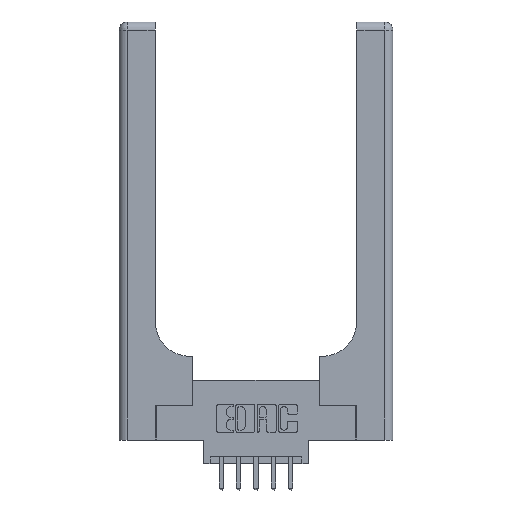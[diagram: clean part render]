
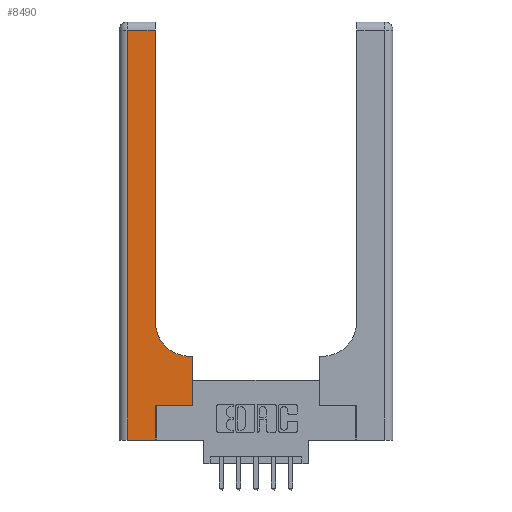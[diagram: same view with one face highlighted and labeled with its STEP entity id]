
A CAD part, top view. The second image highlights one B-rep face of the part: STEP entity #8490.
In plain terms, the highlighted planar face has unit normal (0, 0, 1).
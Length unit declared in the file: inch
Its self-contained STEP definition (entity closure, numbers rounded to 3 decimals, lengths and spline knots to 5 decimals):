
#229 = VERTEX_POINT ( 'NONE', #4516 ) ;
#264 = CARTESIAN_POINT ( 'NONE',  ( 0.265, 0., 0.37 ) ) ;
#535 = CARTESIAN_POINT ( 'NONE',  ( 0.06, 2.94, 0.37 ) ) ;
#684 = EDGE_CURVE ( 'NONE', #13759, #13767, #4708, .T. ) ;
#836 = DIRECTION ( 'NONE',  ( 0., 0., -1. ) ) ;
#930 = CARTESIAN_POINT ( 'NONE',  ( 0.26, 3., 0.37 ) ) ;
#999 = CARTESIAN_POINT ( 'NONE',  ( 0.06, 3., 0.37 ) ) ;
#1139 = VERTEX_POINT ( 'NONE', #5808 ) ;
#1253 = VECTOR ( 'NONE', #1287, 39.37008 ) ;
#1287 = DIRECTION ( 'NONE',  ( -1., 0., 0. ) ) ;
#1362 = CARTESIAN_POINT ( 'NONE',  ( 0.26, 0.6, 0.37 ) ) ;
#1393 = EDGE_CURVE ( 'NONE', #5581, #1139, #13843, .T. ) ;
#2218 = VECTOR ( 'NONE', #6443, 39.37008 ) ;
#2433 = VECTOR ( 'NONE', #2627, 39.37008 ) ;
#2560 = LINE ( 'NONE', #2629, #2978 ) ;
#2594 = LINE ( 'NONE', #6953, #7939 ) ;
#2627 = DIRECTION ( 'NONE',  ( 1., 0., 0. ) ) ;
#2629 = CARTESIAN_POINT ( 'NONE',  ( 0.528, 0.25, 0.37 ) ) ;
#2834 = VECTOR ( 'NONE', #10107, 39.37008 ) ;
#2870 = ORIENTED_EDGE ( 'NONE', *, *, #9795, .T. ) ;
#2978 = VECTOR ( 'NONE', #4777, 39.37008 ) ;
#3374 = VECTOR ( 'NONE', #12914, 39.37008 ) ;
#3708 = CARTESIAN_POINT ( 'NONE',  ( 0.265, 0.25, 0.37 ) ) ;
#4143 = CARTESIAN_POINT ( 'NONE',  ( 0.51, 0.85, 0.37 ) ) ;
#4402 = CARTESIAN_POINT ( 'NONE',  ( 0., 0., 0.37 ) ) ;
#4435 = CARTESIAN_POINT ( 'NONE',  ( 0., 3., 0.37 ) ) ;
#4464 = LINE ( 'NONE', #4402, #10643 ) ;
#4466 = CARTESIAN_POINT ( 'NONE',  ( 0.26, 2.94, 0.37 ) ) ;
#4516 = CARTESIAN_POINT ( 'NONE',  ( 0.528, 0.25, 0.37 ) ) ;
#4708 = LINE ( 'NONE', #1362, #1253 ) ;
#4777 = DIRECTION ( 'NONE',  ( 0., 1., 0. ) ) ;
#5541 = CARTESIAN_POINT ( 'NONE',  ( 0.51, 0.6, 0.37 ) ) ;
#5581 = VERTEX_POINT ( 'NONE', #8639 ) ;
#5808 = CARTESIAN_POINT ( 'NONE',  ( 0.265, 0.25, 0.37 ) ) ;
#6438 = PLANE ( 'NONE',  #11769 ) ;
#6443 = DIRECTION ( 'NONE',  ( 0., 1., 0. ) ) ;
#6792 = AXIS2_PLACEMENT_3D ( 'NONE', #4143, #836, #13835 ) ;
#6953 = CARTESIAN_POINT ( 'NONE',  ( 0., 2.94, 0.37 ) ) ;
#7097 = DIRECTION ( 'NONE',  ( -1., 0., 0. ) ) ;
#7404 = ORIENTED_EDGE ( 'NONE', *, *, #1393, .T. ) ;
#7445 = CIRCLE ( 'NONE', #6792, 0.25 ) ;
#7471 = EDGE_CURVE ( 'NONE', #1139, #229, #13470, .T. ) ;
#7489 = EDGE_CURVE ( 'NONE', #13767, #8089, #7445, .T. ) ;
#7701 = FACE_OUTER_BOUND ( 'NONE', #12515, .T. ) ;
#7719 = CARTESIAN_POINT ( 'NONE',  ( 0.528, 0.6, 0.37 ) ) ;
#7931 = ORIENTED_EDGE ( 'NONE', *, *, #10872, .T. ) ;
#7939 = VECTOR ( 'NONE', #7097, 39.37008 ) ;
#8089 = VERTEX_POINT ( 'NONE', #13291 ) ;
#8354 = VERTEX_POINT ( 'NONE', #9433 ) ;
#8490 = ADVANCED_FACE ( 'NONE', ( #7701 ), #6438, .F. ) ;
#8639 = CARTESIAN_POINT ( 'NONE',  ( 0.265, 0., 0.37 ) ) ;
#8767 = DIRECTION ( 'NONE',  ( 0., 0., -1. ) ) ;
#8933 = ORIENTED_EDGE ( 'NONE', *, *, #7471, .T. ) ;
#9433 = CARTESIAN_POINT ( 'NONE',  ( 0.06, 0., 0.37 ) ) ;
#9557 = EDGE_CURVE ( 'NONE', #8354, #5581, #4464, .T. ) ;
#9767 = LINE ( 'NONE', #930, #2218 ) ;
#9792 = EDGE_CURVE ( 'NONE', #8089, #13301, #9767, .T. ) ;
#9795 = EDGE_CURVE ( 'NONE', #10459, #8354, #9839, .T. ) ;
#9839 = LINE ( 'NONE', #999, #3374 ) ;
#9863 = ORIENTED_EDGE ( 'NONE', *, *, #9792, .T. ) ;
#10107 = DIRECTION ( 'NONE',  ( 0., 1., 0. ) ) ;
#10459 = VERTEX_POINT ( 'NONE', #535 ) ;
#10643 = VECTOR ( 'NONE', #12414, 39.37008 ) ;
#10872 = EDGE_CURVE ( 'NONE', #13301, #10459, #2594, .T. ) ;
#10958 = ORIENTED_EDGE ( 'NONE', *, *, #684, .T. ) ;
#11683 = ORIENTED_EDGE ( 'NONE', *, *, #9557, .T. ) ;
#11769 = AXIS2_PLACEMENT_3D ( 'NONE', #4435, #8767, #13989 ) ;
#12076 = ORIENTED_EDGE ( 'NONE', *, *, #7489, .T. ) ;
#12414 = DIRECTION ( 'NONE',  ( 1., 0., 0. ) ) ;
#12502 = EDGE_CURVE ( 'NONE', #229, #13759, #2560, .T. ) ;
#12515 = EDGE_LOOP ( 'NONE', ( #9863, #7931, #2870, #11683, #7404, #8933, #12686, #10958, #12076 ) ) ;
#12686 = ORIENTED_EDGE ( 'NONE', *, *, #12502, .T. ) ;
#12914 = DIRECTION ( 'NONE',  ( 0., -1., 0. ) ) ;
#13291 = CARTESIAN_POINT ( 'NONE',  ( 0.26, 0.85, 0.37 ) ) ;
#13301 = VERTEX_POINT ( 'NONE', #4466 ) ;
#13470 = LINE ( 'NONE', #3708, #2433 ) ;
#13759 = VERTEX_POINT ( 'NONE', #7719 ) ;
#13767 = VERTEX_POINT ( 'NONE', #5541 ) ;
#13835 = DIRECTION ( 'NONE',  ( 1., 0., 0. ) ) ;
#13843 = LINE ( 'NONE', #264, #2834 ) ;
#13989 = DIRECTION ( 'NONE',  ( -1., 0., 0. ) ) ;
